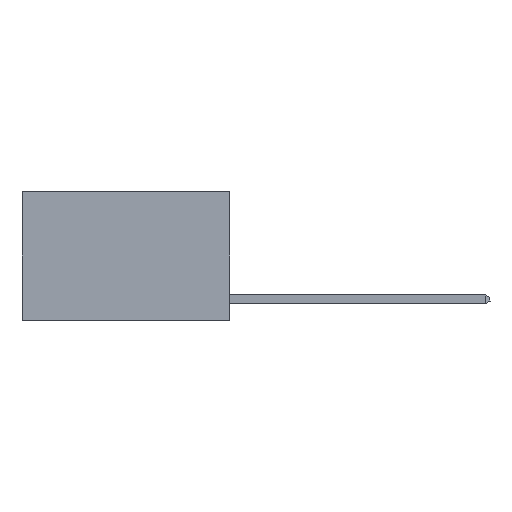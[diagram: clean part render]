
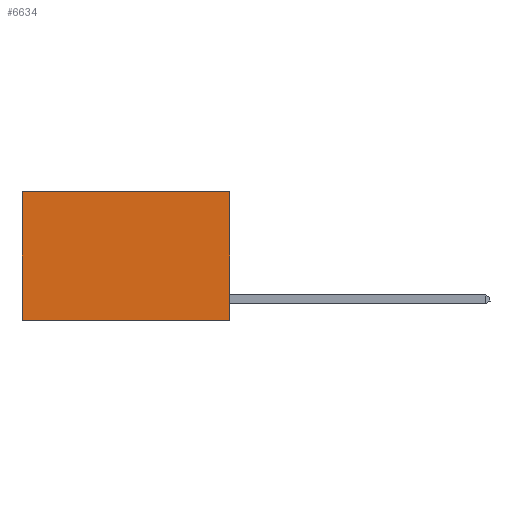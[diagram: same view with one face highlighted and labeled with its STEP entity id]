
A CAD part, left-side view. The second image highlights one B-rep face of the part: STEP entity #6634.
In plain terms, the highlighted planar face has unit normal (-1, 0, 0).
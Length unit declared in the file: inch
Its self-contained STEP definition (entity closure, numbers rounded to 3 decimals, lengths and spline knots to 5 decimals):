
#127 = EDGE_CURVE ( 'NONE', #6339, #5129, #5279, .T. ) ;
#212 = VECTOR ( 'NONE', #10524, 39.37008 ) ;
#504 = CARTESIAN_POINT ( 'NONE',  ( 0.2625, 0., 0. ) ) ;
#572 = DIRECTION ( 'NONE',  ( 0., 1., 0. ) ) ;
#1655 = CARTESIAN_POINT ( 'NONE',  ( 0.2625, 0., -0.37 ) ) ;
#1926 = CARTESIAN_POINT ( 'NONE',  ( 0.2625, 0., 0. ) ) ;
#2400 = LINE ( 'NONE', #11363, #5986 ) ;
#3780 = ORIENTED_EDGE ( 'NONE', *, *, #7571, .F. ) ;
#5097 = ORIENTED_EDGE ( 'NONE', *, *, #11490, .T. ) ;
#5129 = VERTEX_POINT ( 'NONE', #10460 ) ;
#5279 = LINE ( 'NONE', #14162, #212 ) ;
#5314 = FACE_OUTER_BOUND ( 'NONE', #5711, .T. ) ;
#5339 = DIRECTION ( 'NONE',  ( 1., 0., 0. ) ) ;
#5666 = AXIS2_PLACEMENT_3D ( 'NONE', #7881, #5339, #6559 ) ;
#5711 = EDGE_LOOP ( 'NONE', ( #5097, #9065, #3780, #11791 ) ) ;
#5986 = VECTOR ( 'NONE', #572, 39.37008 ) ;
#6339 = VERTEX_POINT ( 'NONE', #1655 ) ;
#6559 = DIRECTION ( 'NONE',  ( 0., 0., -1. ) ) ;
#6634 = ADVANCED_FACE ( 'NONE', ( #5314 ), #12345, .F. ) ;
#6837 = VERTEX_POINT ( 'NONE', #1926 ) ;
#7571 = EDGE_CURVE ( 'NONE', #6837, #6339, #11497, .T. ) ;
#7881 = CARTESIAN_POINT ( 'NONE',  ( 0.2625, 0., 0. ) ) ;
#7882 = DIRECTION ( 'NONE',  ( 0., 0., -1. ) ) ;
#8182 = VECTOR ( 'NONE', #11434, 39.37008 ) ;
#8912 = CARTESIAN_POINT ( 'NONE',  ( 0.2625, 0.6, 0. ) ) ;
#9065 = ORIENTED_EDGE ( 'NONE', *, *, #127, .F. ) ;
#9258 = VERTEX_POINT ( 'NONE', #12008 ) ;
#9545 = EDGE_CURVE ( 'NONE', #6837, #9258, #2400, .T. ) ;
#10460 = CARTESIAN_POINT ( 'NONE',  ( 0.2625, 0.6, -0.37 ) ) ;
#10524 = DIRECTION ( 'NONE',  ( 0., 1., 0. ) ) ;
#11363 = CARTESIAN_POINT ( 'NONE',  ( 0.2625, 0., 0. ) ) ;
#11366 = LINE ( 'NONE', #8912, #8182 ) ;
#11434 = DIRECTION ( 'NONE',  ( 0., 0., -1. ) ) ;
#11490 = EDGE_CURVE ( 'NONE', #9258, #5129, #11366, .T. ) ;
#11497 = LINE ( 'NONE', #504, #11872 ) ;
#11791 = ORIENTED_EDGE ( 'NONE', *, *, #9545, .T. ) ;
#11872 = VECTOR ( 'NONE', #7882, 39.37008 ) ;
#12008 = CARTESIAN_POINT ( 'NONE',  ( 0.2625, 0.6, 0. ) ) ;
#12345 = PLANE ( 'NONE',  #5666 ) ;
#14162 = CARTESIAN_POINT ( 'NONE',  ( 0.2625, 0., -0.37 ) ) ;
